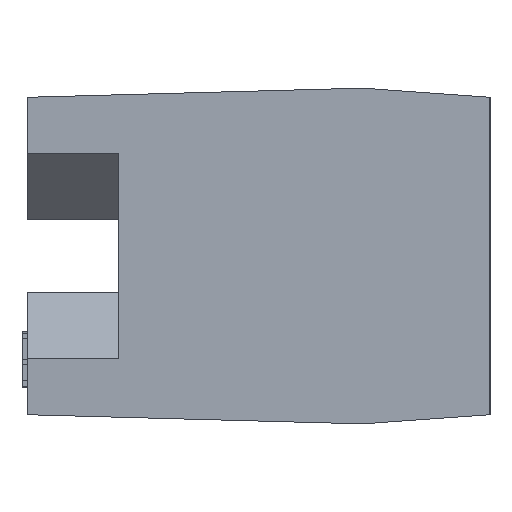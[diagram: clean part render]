
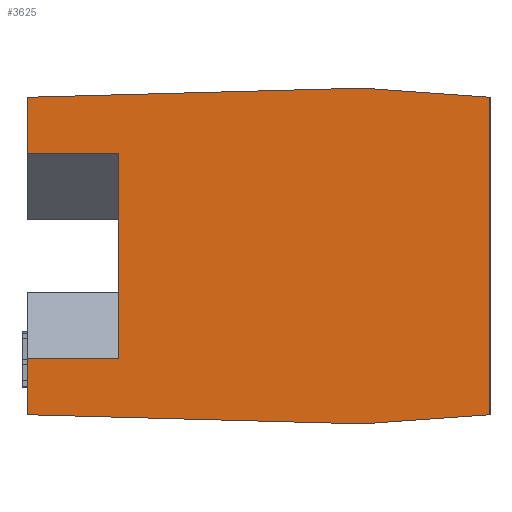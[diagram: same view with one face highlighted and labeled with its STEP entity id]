
A CAD part, left-side view. The second image highlights one B-rep face of the part: STEP entity #3625.
In plain terms, the highlighted planar face has unit normal (-1, 0, 0).
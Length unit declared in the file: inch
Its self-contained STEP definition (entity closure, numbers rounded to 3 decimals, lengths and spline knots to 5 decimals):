
#272 = ORIENTED_EDGE ( 'NONE', *, *, #8997, .F. ) ;
#374 = VECTOR ( 'NONE', #5978, 39.37008 ) ;
#412 = CARTESIAN_POINT ( 'NONE',  ( -4.5, 0.365, -0.1005 ) ) ;
#700 = CARTESIAN_POINT ( 'NONE',  ( -4.5, 0.365, 0.1005 ) ) ;
#739 = CARTESIAN_POINT ( 'NONE',  ( -4.5, 0.365, -0.1005 ) ) ;
#838 = ORIENTED_EDGE ( 'NONE', *, *, #3953, .F. ) ;
#901 = VERTEX_POINT ( 'NONE', #8538 ) ;
#1455 = CARTESIAN_POINT ( 'NONE',  ( -4.5, 0.455, -0.156 ) ) ;
#1556 = EDGE_CURVE ( 'NONE', #9358, #3136, #8376, .T. ) ;
#1841 = CARTESIAN_POINT ( 'NONE',  ( -4.5, 0.455, -0.1005 ) ) ;
#2100 = LINE ( 'NONE', #5220, #7218 ) ;
#2459 = CARTESIAN_POINT ( 'NONE',  ( -4.5, 0.125, 0.165 ) ) ;
#2533 = DIRECTION ( 'NONE',  ( 0., 0., 1. ) ) ;
#2615 = LINE ( 'NONE', #739, #11595 ) ;
#2649 = EDGE_CURVE ( 'NONE', #901, #6997, #4441, .T. ) ;
#2683 = DIRECTION ( 'NONE',  ( 0., 1., 0. ) ) ;
#2693 = VERTEX_POINT ( 'NONE', #1841 ) ;
#2774 = ORIENTED_EDGE ( 'NONE', *, *, #2649, .T. ) ;
#3035 = DIRECTION ( 'NONE',  ( 0., 1., 0. ) ) ;
#3055 = CARTESIAN_POINT ( 'NONE',  ( -4.5, 0.455, -0.156 ) ) ;
#3078 = EDGE_LOOP ( 'NONE', ( #8284, #6065, #5072, #5987, #2774, #8270, #6292, #7987, #272, #838 ) ) ;
#3136 = VERTEX_POINT ( 'NONE', #12473 ) ;
#3471 = CARTESIAN_POINT ( 'NONE',  ( -4.5, 0.125, -0.165 ) ) ;
#3559 = DIRECTION ( 'NONE',  ( 0., 1., -0.027 ) ) ;
#3566 = EDGE_CURVE ( 'NONE', #5965, #10566, #11338, .T. ) ;
#3625 = ADVANCED_FACE ( 'NONE', ( #9505 ), #7426, .F. ) ;
#3734 = VERTEX_POINT ( 'NONE', #8909 ) ;
#3914 = EDGE_CURVE ( 'NONE', #6997, #9358, #7012, .T. ) ;
#3953 = EDGE_CURVE ( 'NONE', #10566, #3734, #11829, .T. ) ;
#4068 = VECTOR ( 'NONE', #6906, 39.37008 ) ;
#4086 = VECTOR ( 'NONE', #10284, 39.37008 ) ;
#4313 = EDGE_CURVE ( 'NONE', #7129, #2693, #2100, .T. ) ;
#4350 = CARTESIAN_POINT ( 'NONE',  ( -4.5, 0.455, 0.156 ) ) ;
#4441 = LINE ( 'NONE', #3471, #4068 ) ;
#4858 = EDGE_CURVE ( 'NONE', #5965, #2693, #2615, .T. ) ;
#4906 = LINE ( 'NONE', #11687, #7246 ) ;
#5072 = ORIENTED_EDGE ( 'NONE', *, *, #4313, .F. ) ;
#5220 = CARTESIAN_POINT ( 'NONE',  ( -4.5, 0.455, -0.156 ) ) ;
#5527 = CARTESIAN_POINT ( 'NONE',  ( -4.5, 0., 0.156 ) ) ;
#5639 = LINE ( 'NONE', #6682, #9843 ) ;
#5766 = DIRECTION ( 'NONE',  ( 0., -1., -0.027 ) ) ;
#5965 = VERTEX_POINT ( 'NONE', #412 ) ;
#5978 = DIRECTION ( 'NONE',  ( 0., 0., 1. ) ) ;
#5987 = ORIENTED_EDGE ( 'NONE', *, *, #7795, .T. ) ;
#6018 = LINE ( 'NONE', #9129, #8832 ) ;
#6065 = ORIENTED_EDGE ( 'NONE', *, *, #4858, .T. ) ;
#6240 = VERTEX_POINT ( 'NONE', #4350 ) ;
#6292 = ORIENTED_EDGE ( 'NONE', *, *, #1556, .T. ) ;
#6682 = CARTESIAN_POINT ( 'NONE',  ( -4.5, 0.455, 0.156 ) ) ;
#6906 = DIRECTION ( 'NONE',  ( 0., -0.997, 0.072 ) ) ;
#6997 = VERTEX_POINT ( 'NONE', #11408 ) ;
#7003 = VECTOR ( 'NONE', #2533, 39.37008 ) ;
#7012 = LINE ( 'NONE', #7911, #374 ) ;
#7129 = VERTEX_POINT ( 'NONE', #3055 ) ;
#7218 = VECTOR ( 'NONE', #11083, 39.37008 ) ;
#7246 = VECTOR ( 'NONE', #5766, 39.37008 ) ;
#7426 = PLANE ( 'NONE',  #11774 ) ;
#7487 = CARTESIAN_POINT ( 'NONE',  ( -4.5, 0.365, -0.1005 ) ) ;
#7795 = EDGE_CURVE ( 'NONE', #7129, #901, #4906, .T. ) ;
#7911 = CARTESIAN_POINT ( 'NONE',  ( -4.5, 0., -0.156 ) ) ;
#7987 = ORIENTED_EDGE ( 'NONE', *, *, #10489, .T. ) ;
#8019 = DIRECTION ( 'NONE',  ( 0., 0., 1. ) ) ;
#8270 = ORIENTED_EDGE ( 'NONE', *, *, #3914, .T. ) ;
#8284 = ORIENTED_EDGE ( 'NONE', *, *, #3566, .F. ) ;
#8334 = DIRECTION ( 'NONE',  ( 1., 0., 0. ) ) ;
#8376 = LINE ( 'NONE', #2459, #4086 ) ;
#8455 = VECTOR ( 'NONE', #3035, 39.37008 ) ;
#8538 = CARTESIAN_POINT ( 'NONE',  ( -4.5, 0.125, -0.165 ) ) ;
#8832 = VECTOR ( 'NONE', #8019, 39.37008 ) ;
#8909 = CARTESIAN_POINT ( 'NONE',  ( -4.5, 0.455, 0.1005 ) ) ;
#8997 = EDGE_CURVE ( 'NONE', #3734, #6240, #6018, .T. ) ;
#9020 = CARTESIAN_POINT ( 'NONE',  ( -4.5, 0.365, 0.1005 ) ) ;
#9129 = CARTESIAN_POINT ( 'NONE',  ( -4.5, 0.455, -0.156 ) ) ;
#9358 = VERTEX_POINT ( 'NONE', #5527 ) ;
#9383 = DIRECTION ( 'NONE',  ( 0., 0., -1. ) ) ;
#9505 = FACE_OUTER_BOUND ( 'NONE', #3078, .T. ) ;
#9843 = VECTOR ( 'NONE', #3559, 39.37008 ) ;
#10284 = DIRECTION ( 'NONE',  ( 0., 0.997, 0.072 ) ) ;
#10489 = EDGE_CURVE ( 'NONE', #3136, #6240, #5639, .T. ) ;
#10566 = VERTEX_POINT ( 'NONE', #700 ) ;
#11083 = DIRECTION ( 'NONE',  ( 0., 0., 1. ) ) ;
#11338 = LINE ( 'NONE', #7487, #7003 ) ;
#11408 = CARTESIAN_POINT ( 'NONE',  ( -4.5, 0., -0.156 ) ) ;
#11595 = VECTOR ( 'NONE', #2683, 39.37008 ) ;
#11687 = CARTESIAN_POINT ( 'NONE',  ( -4.5, 0.455, -0.156 ) ) ;
#11774 = AXIS2_PLACEMENT_3D ( 'NONE', #1455, #8334, #9383 ) ;
#11829 = LINE ( 'NONE', #9020, #8455 ) ;
#12473 = CARTESIAN_POINT ( 'NONE',  ( -4.5, 0.125, 0.165 ) ) ;
